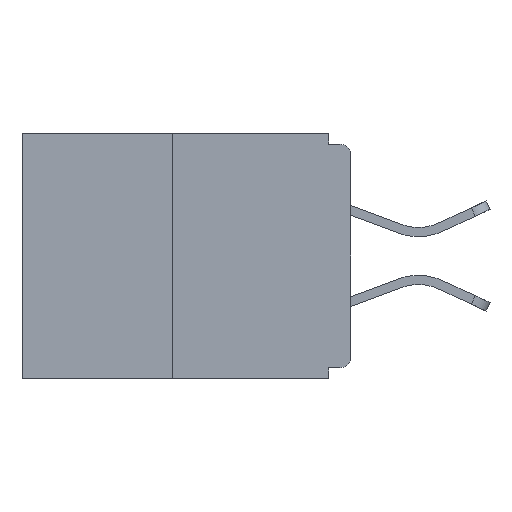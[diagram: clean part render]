
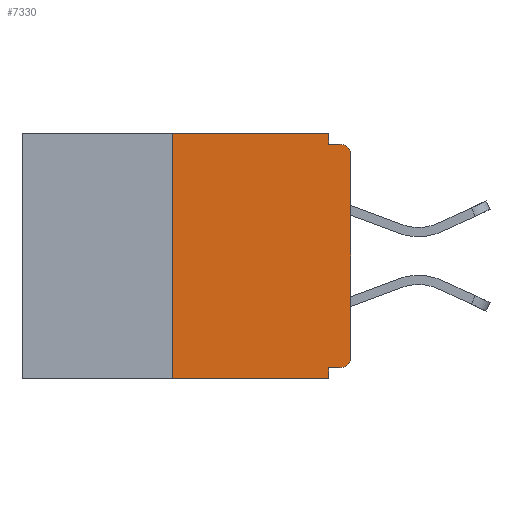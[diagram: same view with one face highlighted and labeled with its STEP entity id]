
A CAD part, left-side view. The second image highlights one B-rep face of the part: STEP entity #7330.
In plain terms, the highlighted planar face has unit normal (-1, 0, 0).
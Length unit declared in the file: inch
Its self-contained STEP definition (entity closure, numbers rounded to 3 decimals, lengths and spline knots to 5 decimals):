
#46 = LINE ( 'NONE', #8827, #807 ) ;
#141 = CARTESIAN_POINT ( 'NONE',  ( 0., 0., -0.313 ) ) ;
#197 = VERTEX_POINT ( 'NONE', #5999 ) ;
#451 = VERTEX_POINT ( 'NONE', #6247 ) ;
#497 = EDGE_CURVE ( 'NONE', #451, #8629, #1783, .T. ) ;
#807 = VECTOR ( 'NONE', #3293, 39.37008 ) ;
#960 = VECTOR ( 'NONE', #2890, 39.37008 ) ;
#968 = CARTESIAN_POINT ( 'NONE',  ( 0., 0.031, 0. ) ) ;
#972 = EDGE_CURVE ( 'NONE', #10311, #3837, #5238, .T. ) ;
#1076 = VECTOR ( 'NONE', #1513, 39.37008 ) ;
#1210 = ORIENTED_EDGE ( 'NONE', *, *, #10472, .F. ) ;
#1513 = DIRECTION ( 'NONE',  ( 0., 0., 1. ) ) ;
#1707 = AXIS2_PLACEMENT_3D ( 'NONE', #1823, #2771, #10496 ) ;
#1766 = VERTEX_POINT ( 'NONE', #11172 ) ;
#1783 = LINE ( 'NONE', #10173, #4639 ) ;
#1823 = CARTESIAN_POINT ( 'NONE',  ( 0., 0.46, 0. ) ) ;
#1882 = ORIENTED_EDGE ( 'NONE', *, *, #2055, .F. ) ;
#2020 = CARTESIAN_POINT ( 'NONE',  ( 0., 0., -0.328 ) ) ;
#2043 = ORIENTED_EDGE ( 'NONE', *, *, #7236, .T. ) ;
#2055 = EDGE_CURVE ( 'NONE', #10311, #451, #7281, .T. ) ;
#2056 = VERTEX_POINT ( 'NONE', #6866 ) ;
#2214 = CARTESIAN_POINT ( 'NONE',  ( 0., 0., -0.015 ) ) ;
#2270 = ORIENTED_EDGE ( 'NONE', *, *, #12472, .F. ) ;
#2411 = DIRECTION ( 'NONE',  ( -1., 0., 0. ) ) ;
#2771 = DIRECTION ( 'NONE',  ( 1., 0., 0. ) ) ;
#2827 = ORIENTED_EDGE ( 'NONE', *, *, #497, .F. ) ;
#2890 = DIRECTION ( 'NONE',  ( 0., -1., 0. ) ) ;
#3067 = ORIENTED_EDGE ( 'NONE', *, *, #7936, .F. ) ;
#3293 = DIRECTION ( 'NONE',  ( 0., 0., -1. ) ) ;
#3426 = ORIENTED_EDGE ( 'NONE', *, *, #8829, .T. ) ;
#3545 = CIRCLE ( 'NONE', #6478, 0.015 ) ;
#3837 = VERTEX_POINT ( 'NONE', #141 ) ;
#4045 = CARTESIAN_POINT ( 'NONE',  ( 0., 0.031, -0.343 ) ) ;
#4301 = CARTESIAN_POINT ( 'NONE',  ( 0., 0.015, -0.03 ) ) ;
#4309 = LINE ( 'NONE', #2214, #8554 ) ;
#4341 = DIRECTION ( 'NONE',  ( 0., 0., -1. ) ) ;
#4639 = VECTOR ( 'NONE', #4341, 39.37008 ) ;
#4765 = PLANE ( 'NONE',  #1707 ) ;
#5238 = CIRCLE ( 'NONE', #11955, 0.015 ) ;
#5241 = ORIENTED_EDGE ( 'NONE', *, *, #6213, .T. ) ;
#5382 = VERTEX_POINT ( 'NONE', #11037 ) ;
#5498 = CARTESIAN_POINT ( 'NONE',  ( 0., 0., 0. ) ) ;
#5521 = DIRECTION ( 'NONE',  ( -1., 0., 0. ) ) ;
#5811 = VERTEX_POINT ( 'NONE', #11751 ) ;
#5999 = CARTESIAN_POINT ( 'NONE',  ( 0., 0., -0.03 ) ) ;
#6052 = DIRECTION ( 'NONE',  ( 0., -1., 0. ) ) ;
#6213 = EDGE_CURVE ( 'NONE', #3837, #197, #11682, .T. ) ;
#6247 = CARTESIAN_POINT ( 'NONE',  ( 0., 0.031, -0.328 ) ) ;
#6403 = CARTESIAN_POINT ( 'NONE',  ( 0., 0.015, -0.313 ) ) ;
#6455 = VERTEX_POINT ( 'NONE', #968 ) ;
#6478 = AXIS2_PLACEMENT_3D ( 'NONE', #4301, #2411, #11051 ) ;
#6707 = CARTESIAN_POINT ( 'NONE',  ( 0., 0.46, -0.343 ) ) ;
#6866 = CARTESIAN_POINT ( 'NONE',  ( 0., 0.25, 0. ) ) ;
#7000 = ORIENTED_EDGE ( 'NONE', *, *, #11725, .F. ) ;
#7111 = LINE ( 'NONE', #8957, #1076 ) ;
#7236 = EDGE_CURVE ( 'NONE', #1766, #8629, #7911, .T. ) ;
#7281 = LINE ( 'NONE', #2020, #12381 ) ;
#7330 = ADVANCED_FACE ( 'NONE', ( #10897 ), #4765, .F. ) ;
#7696 = VECTOR ( 'NONE', #12174, 39.37008 ) ;
#7911 = LINE ( 'NONE', #6707, #960 ) ;
#7936 = EDGE_CURVE ( 'NONE', #5811, #5382, #4309, .T. ) ;
#8043 = ORIENTED_EDGE ( 'NONE', *, *, #972, .T. ) ;
#8554 = VECTOR ( 'NONE', #6052, 39.37008 ) ;
#8629 = VERTEX_POINT ( 'NONE', #4045 ) ;
#8665 = CARTESIAN_POINT ( 'NONE',  ( 0., 0.015, -0.328 ) ) ;
#8827 = CARTESIAN_POINT ( 'NONE',  ( 0., 0.031, 0. ) ) ;
#8829 = EDGE_CURVE ( 'NONE', #197, #5382, #3545, .T. ) ;
#8957 = CARTESIAN_POINT ( 'NONE',  ( 0., 0.25, 0. ) ) ;
#9292 = CARTESIAN_POINT ( 'NONE',  ( 0., 0.46, 0. ) ) ;
#9348 = EDGE_LOOP ( 'NONE', ( #2270, #7000, #2043, #2827, #1882, #8043, #5241, #3426, #3067, #1210 ) ) ;
#9583 = VECTOR ( 'NONE', #11223, 39.37008 ) ;
#9652 = DIRECTION ( 'NONE',  ( 0., 1., 0. ) ) ;
#10173 = CARTESIAN_POINT ( 'NONE',  ( 0., 0.031, -0.343 ) ) ;
#10311 = VERTEX_POINT ( 'NONE', #8665 ) ;
#10472 = EDGE_CURVE ( 'NONE', #6455, #5811, #46, .T. ) ;
#10496 = DIRECTION ( 'NONE',  ( 0., 0., -1. ) ) ;
#10663 = LINE ( 'NONE', #9292, #7696 ) ;
#10897 = FACE_OUTER_BOUND ( 'NONE', #9348, .T. ) ;
#11037 = CARTESIAN_POINT ( 'NONE',  ( 0., 0.015, -0.015 ) ) ;
#11051 = DIRECTION ( 'NONE',  ( 0., 0., -1. ) ) ;
#11172 = CARTESIAN_POINT ( 'NONE',  ( 0., 0.25, -0.343 ) ) ;
#11223 = DIRECTION ( 'NONE',  ( 0., 0., 1. ) ) ;
#11682 = LINE ( 'NONE', #5498, #9583 ) ;
#11725 = EDGE_CURVE ( 'NONE', #1766, #2056, #7111, .T. ) ;
#11751 = CARTESIAN_POINT ( 'NONE',  ( 0., 0.031, -0.015 ) ) ;
#11955 = AXIS2_PLACEMENT_3D ( 'NONE', #6403, #5521, #12239 ) ;
#12174 = DIRECTION ( 'NONE',  ( 0., -1., 0. ) ) ;
#12239 = DIRECTION ( 'NONE',  ( 0., 0., -1. ) ) ;
#12381 = VECTOR ( 'NONE', #9652, 39.37008 ) ;
#12472 = EDGE_CURVE ( 'NONE', #2056, #6455, #10663, .T. ) ;
